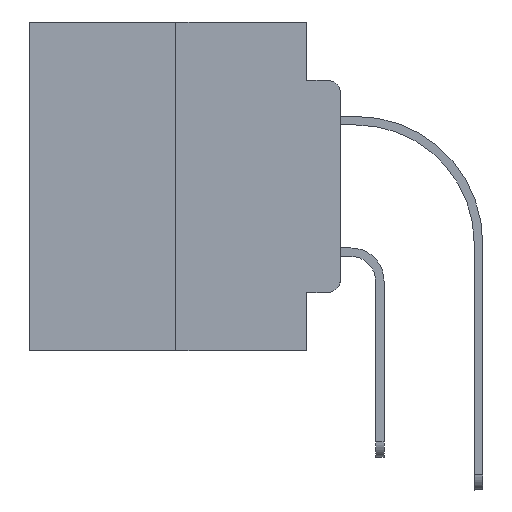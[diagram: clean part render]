
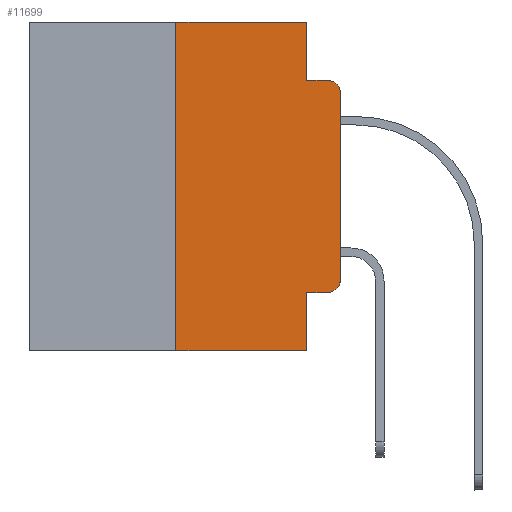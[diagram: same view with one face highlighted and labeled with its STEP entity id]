
A CAD part, left-side view. The second image highlights one B-rep face of the part: STEP entity #11699.
In plain terms, the highlighted planar face has unit normal (-1, 0, 0).
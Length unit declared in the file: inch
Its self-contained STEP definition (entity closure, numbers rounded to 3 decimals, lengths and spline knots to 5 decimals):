
#80 = CARTESIAN_POINT ( 'NONE',  ( 0., 0.25, 0. ) ) ;
#157 = CARTESIAN_POINT ( 'NONE',  ( 0., 0., -0.3915 ) ) ;
#510 = DIRECTION ( 'NONE',  ( 0., 0., 1. ) ) ;
#775 = CARTESIAN_POINT ( 'NONE',  ( 0., 0.25, 0. ) ) ;
#867 = EDGE_CURVE ( 'NONE', #22842, #12405, #20003, .T. ) ;
#1089 = DIRECTION ( 'NONE',  ( 0., 0., -1. ) ) ;
#1271 = DIRECTION ( 'NONE',  ( -1., 0., 0. ) ) ;
#1426 = EDGE_CURVE ( 'NONE', #16414, #4786, #21995, .T. ) ;
#1550 = CARTESIAN_POINT ( 'NONE',  ( 0., 0.02, -0.1085 ) ) ;
#1949 = EDGE_CURVE ( 'NONE', #15050, #16414, #7927, .T. ) ;
#1986 = VERTEX_POINT ( 'NONE', #25540 ) ;
#2273 = EDGE_CURVE ( 'NONE', #22842, #10643, #20266, .T. ) ;
#2725 = CARTESIAN_POINT ( 'NONE',  ( 0., 0.473, 0. ) ) ;
#3134 = EDGE_CURVE ( 'NONE', #11561, #15050, #16765, .T. ) ;
#3576 = AXIS2_PLACEMENT_3D ( 'NONE', #16335, #12214, #1089 ) ;
#3659 = CARTESIAN_POINT ( 'NONE',  ( 0., 0.051, -0.4115 ) ) ;
#3815 = AXIS2_PLACEMENT_3D ( 'NONE', #1550, #1271, #5392 ) ;
#3903 = DIRECTION ( 'NONE',  ( 0., 0., -1. ) ) ;
#4044 = AXIS2_PLACEMENT_3D ( 'NONE', #2725, #7274, #4681 ) ;
#4319 = ORIENTED_EDGE ( 'NONE', *, *, #10481, .F. ) ;
#4681 = DIRECTION ( 'NONE',  ( 0., 0., -1. ) ) ;
#4786 = VERTEX_POINT ( 'NONE', #26232 ) ;
#4787 = ORIENTED_EDGE ( 'NONE', *, *, #3134, .T. ) ;
#4820 = FACE_OUTER_BOUND ( 'NONE', #5066, .T. ) ;
#5066 = EDGE_LOOP ( 'NONE', ( #20398, #22745, #11801, #5394, #4319, #19237, #24999, #19252, #24416, #4787 ) ) ;
#5123 = LINE ( 'NONE', #16093, #5741 ) ;
#5392 = DIRECTION ( 'NONE',  ( 0., 0., -1. ) ) ;
#5394 = ORIENTED_EDGE ( 'NONE', *, *, #27831, .F. ) ;
#5741 = VECTOR ( 'NONE', #13819, 39.37008 ) ;
#7274 = DIRECTION ( 'NONE',  ( 1., 0., 0. ) ) ;
#7706 = VERTEX_POINT ( 'NONE', #3659 ) ;
#7927 = LINE ( 'NONE', #12210, #18958 ) ;
#8612 = VERTEX_POINT ( 'NONE', #13666 ) ;
#8634 = DIRECTION ( 'NONE',  ( 0., -1., 0. ) ) ;
#9407 = LINE ( 'NONE', #24067, #24928 ) ;
#10481 = EDGE_CURVE ( 'NONE', #10643, #8612, #27252, .T. ) ;
#10491 = CARTESIAN_POINT ( 'NONE',  ( 0., 0.051, 0. ) ) ;
#10643 = VERTEX_POINT ( 'NONE', #80 ) ;
#11561 = VERTEX_POINT ( 'NONE', #18943 ) ;
#11636 = EDGE_CURVE ( 'NONE', #7706, #12405, #9407, .T. ) ;
#11699 = ADVANCED_FACE ( 'NONE', ( #4820 ), #21802, .F. ) ;
#11801 = ORIENTED_EDGE ( 'NONE', *, *, #28002, .F. ) ;
#12210 = CARTESIAN_POINT ( 'NONE',  ( 0., 0., 0. ) ) ;
#12214 = DIRECTION ( 'NONE',  ( -1., 0., 0. ) ) ;
#12405 = VERTEX_POINT ( 'NONE', #27607 ) ;
#13666 = CARTESIAN_POINT ( 'NONE',  ( 0., 0.051, 0. ) ) ;
#13819 = DIRECTION ( 'NONE',  ( 0., -1., 0. ) ) ;
#13908 = DIRECTION ( 'NONE',  ( 0., 0., 1. ) ) ;
#14717 = CARTESIAN_POINT ( 'NONE',  ( 0., 0., -0.1085 ) ) ;
#14793 = VECTOR ( 'NONE', #19580, 39.37008 ) ;
#15050 = VERTEX_POINT ( 'NONE', #157 ) ;
#16093 = CARTESIAN_POINT ( 'NONE',  ( 0., 0.051, -0.4115 ) ) ;
#16335 = CARTESIAN_POINT ( 'NONE',  ( 0., 0.02, -0.3915 ) ) ;
#16414 = VERTEX_POINT ( 'NONE', #14717 ) ;
#16765 = CIRCLE ( 'NONE', #3576, 0.02 ) ;
#17636 = EDGE_CURVE ( 'NONE', #7706, #11561, #5123, .T. ) ;
#17758 = VECTOR ( 'NONE', #3903, 39.37008 ) ;
#18117 = VECTOR ( 'NONE', #510, 39.37008 ) ;
#18244 = CARTESIAN_POINT ( 'NONE',  ( 0., 0.25, -0.5 ) ) ;
#18861 = DIRECTION ( 'NONE',  ( 0., -1., 0. ) ) ;
#18943 = CARTESIAN_POINT ( 'NONE',  ( 0., 0.02, -0.4115 ) ) ;
#18958 = VECTOR ( 'NONE', #13908, 39.37008 ) ;
#19237 = ORIENTED_EDGE ( 'NONE', *, *, #2273, .F. ) ;
#19252 = ORIENTED_EDGE ( 'NONE', *, *, #11636, .F. ) ;
#19580 = DIRECTION ( 'NONE',  ( 0., -1., 0. ) ) ;
#19695 = LINE ( 'NONE', #26488, #26931 ) ;
#20003 = LINE ( 'NONE', #26500, #14793 ) ;
#20266 = LINE ( 'NONE', #775, #18117 ) ;
#20398 = ORIENTED_EDGE ( 'NONE', *, *, #1949, .T. ) ;
#20996 = LINE ( 'NONE', #10491, #17758 ) ;
#21730 = VECTOR ( 'NONE', #18861, 39.37008 ) ;
#21802 = PLANE ( 'NONE',  #4044 ) ;
#21995 = CIRCLE ( 'NONE', #3815, 0.02 ) ;
#22745 = ORIENTED_EDGE ( 'NONE', *, *, #1426, .T. ) ;
#22842 = VERTEX_POINT ( 'NONE', #18244 ) ;
#24067 = CARTESIAN_POINT ( 'NONE',  ( 0., 0.051, 0. ) ) ;
#24416 = ORIENTED_EDGE ( 'NONE', *, *, #17636, .T. ) ;
#24928 = VECTOR ( 'NONE', #26309, 39.37008 ) ;
#24986 = CARTESIAN_POINT ( 'NONE',  ( 0., 0.473, 0. ) ) ;
#24999 = ORIENTED_EDGE ( 'NONE', *, *, #867, .T. ) ;
#25540 = CARTESIAN_POINT ( 'NONE',  ( 0., 0.051, -0.0885 ) ) ;
#26232 = CARTESIAN_POINT ( 'NONE',  ( 0., 0.02, -0.0885 ) ) ;
#26309 = DIRECTION ( 'NONE',  ( 0., 0., -1. ) ) ;
#26488 = CARTESIAN_POINT ( 'NONE',  ( 0., 0.051, -0.0885 ) ) ;
#26500 = CARTESIAN_POINT ( 'NONE',  ( 0., 0.473, -0.5 ) ) ;
#26931 = VECTOR ( 'NONE', #8634, 39.37008 ) ;
#27252 = LINE ( 'NONE', #24986, #21730 ) ;
#27607 = CARTESIAN_POINT ( 'NONE',  ( 0., 0.051, -0.5 ) ) ;
#27831 = EDGE_CURVE ( 'NONE', #8612, #1986, #20996, .T. ) ;
#28002 = EDGE_CURVE ( 'NONE', #1986, #4786, #19695, .T. ) ;
